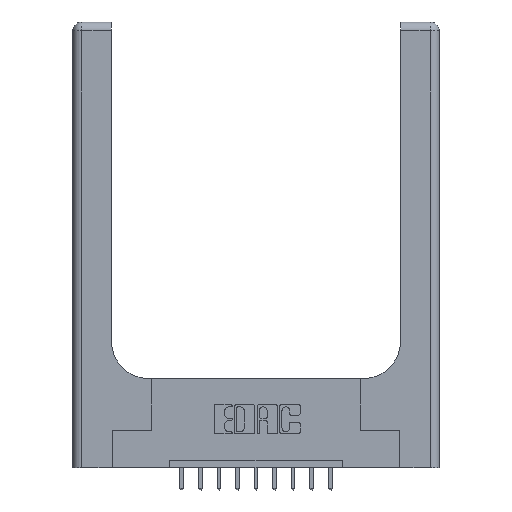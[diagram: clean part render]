
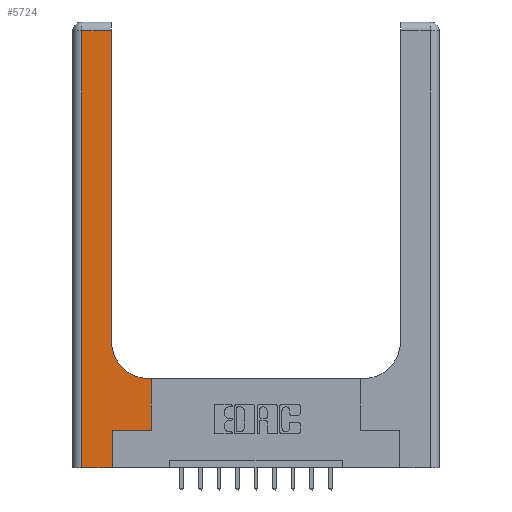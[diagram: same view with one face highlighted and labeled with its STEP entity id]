
A CAD part, top view. The second image highlights one B-rep face of the part: STEP entity #5724.
In plain terms, the highlighted planar face has unit normal (0, 0, 1).
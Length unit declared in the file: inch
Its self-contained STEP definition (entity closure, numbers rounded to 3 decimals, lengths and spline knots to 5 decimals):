
#124 = CARTESIAN_POINT ( 'NONE',  ( 0.528, 0.25, 0.37 ) ) ;
#149 = DIRECTION ( 'NONE',  ( 1., 0., 0. ) ) ;
#223 = CARTESIAN_POINT ( 'NONE',  ( 0.51, 0.85, 0.37 ) ) ;
#633 = DIRECTION ( 'NONE',  ( 0., 1., 0. ) ) ;
#662 = LINE ( 'NONE', #5479, #15247 ) ;
#711 = LINE ( 'NONE', #15052, #2263 ) ;
#1183 = LINE ( 'NONE', #14420, #14164 ) ;
#1320 = EDGE_CURVE ( 'NONE', #15670, #12019, #7495, .T. ) ;
#1458 = CARTESIAN_POINT ( 'NONE',  ( 0.26, 0.6, 0.37 ) ) ;
#1484 = VECTOR ( 'NONE', #2648, 39.37008 ) ;
#1538 = CARTESIAN_POINT ( 'NONE',  ( 0.265, 0.25, 0.37 ) ) ;
#1796 = ORIENTED_EDGE ( 'NONE', *, *, #11131, .T. ) ;
#2263 = VECTOR ( 'NONE', #633, 39.37008 ) ;
#2351 = EDGE_LOOP ( 'NONE', ( #15493, #11900, #12469, #4827, #13636, #3973, #2980, #12693, #1796 ) ) ;
#2383 = LINE ( 'NONE', #11051, #11143 ) ;
#2530 = VECTOR ( 'NONE', #12328, 39.37008 ) ;
#2648 = DIRECTION ( 'NONE',  ( 0., 1., 0. ) ) ;
#2891 = VERTEX_POINT ( 'NONE', #4877 ) ;
#2980 = ORIENTED_EDGE ( 'NONE', *, *, #1320, .T. ) ;
#3057 = DIRECTION ( 'NONE',  ( 0., 0., -1. ) ) ;
#3136 = DIRECTION ( 'NONE',  ( -1., 0., 0. ) ) ;
#3211 = FACE_OUTER_BOUND ( 'NONE', #2351, .T. ) ;
#3316 = EDGE_CURVE ( 'NONE', #12019, #2891, #11160, .T. ) ;
#3808 = AXIS2_PLACEMENT_3D ( 'NONE', #223, #11268, #149 ) ;
#3973 = ORIENTED_EDGE ( 'NONE', *, *, #5470, .T. ) ;
#4302 = CARTESIAN_POINT ( 'NONE',  ( 0.528, 0.25, 0.37 ) ) ;
#4585 = VERTEX_POINT ( 'NONE', #13779 ) ;
#4628 = VERTEX_POINT ( 'NONE', #14381 ) ;
#4827 = ORIENTED_EDGE ( 'NONE', *, *, #6338, .T. ) ;
#4877 = CARTESIAN_POINT ( 'NONE',  ( 0.51, 0.6, 0.37 ) ) ;
#5319 = CARTESIAN_POINT ( 'NONE',  ( 0.265, 0., 0.37 ) ) ;
#5470 = EDGE_CURVE ( 'NONE', #12850, #15670, #1183, .T. ) ;
#5479 = CARTESIAN_POINT ( 'NONE',  ( 0.06, 3., 0.37 ) ) ;
#5724 = ADVANCED_FACE ( 'NONE', ( #3211 ), #8146, .F. ) ;
#6338 = EDGE_CURVE ( 'NONE', #4628, #4585, #2383, .T. ) ;
#7105 = EDGE_CURVE ( 'NONE', #11960, #7735, #14673, .T. ) ;
#7495 = LINE ( 'NONE', #124, #1484 ) ;
#7673 = AXIS2_PLACEMENT_3D ( 'NONE', #11731, #3057, #3136 ) ;
#7735 = VERTEX_POINT ( 'NONE', #9636 ) ;
#7780 = CARTESIAN_POINT ( 'NONE',  ( 0.528, 0.6, 0.37 ) ) ;
#7884 = VECTOR ( 'NONE', #10253, 39.37008 ) ;
#8146 = PLANE ( 'NONE',  #7673 ) ;
#8441 = EDGE_CURVE ( 'NONE', #4585, #12850, #9130, .T. ) ;
#8839 = EDGE_CURVE ( 'NONE', #12697, #11960, #711, .T. ) ;
#9130 = LINE ( 'NONE', #5319, #7884 ) ;
#9636 = CARTESIAN_POINT ( 'NONE',  ( 0.06, 2.94, 0.37 ) ) ;
#9824 = DIRECTION ( 'NONE',  ( 1., 0., 0. ) ) ;
#10253 = DIRECTION ( 'NONE',  ( 0., 1., 0. ) ) ;
#10330 = DIRECTION ( 'NONE',  ( 0., -1., 0. ) ) ;
#11051 = CARTESIAN_POINT ( 'NONE',  ( 0., 0., 0.37 ) ) ;
#11131 = EDGE_CURVE ( 'NONE', #2891, #12697, #13231, .T. ) ;
#11143 = VECTOR ( 'NONE', #13429, 39.37008 ) ;
#11160 = LINE ( 'NONE', #1458, #14305 ) ;
#11268 = DIRECTION ( 'NONE',  ( 0., 0., -1. ) ) ;
#11731 = CARTESIAN_POINT ( 'NONE',  ( 0., 3., 0.37 ) ) ;
#11827 = EDGE_CURVE ( 'NONE', #7735, #4628, #662, .T. ) ;
#11900 = ORIENTED_EDGE ( 'NONE', *, *, #7105, .T. ) ;
#11960 = VERTEX_POINT ( 'NONE', #14977 ) ;
#12019 = VERTEX_POINT ( 'NONE', #7780 ) ;
#12328 = DIRECTION ( 'NONE',  ( -1., 0., 0. ) ) ;
#12354 = DIRECTION ( 'NONE',  ( -1., 0., 0. ) ) ;
#12407 = CARTESIAN_POINT ( 'NONE',  ( 0., 2.94, 0.37 ) ) ;
#12469 = ORIENTED_EDGE ( 'NONE', *, *, #11827, .T. ) ;
#12693 = ORIENTED_EDGE ( 'NONE', *, *, #3316, .T. ) ;
#12697 = VERTEX_POINT ( 'NONE', #15419 ) ;
#12850 = VERTEX_POINT ( 'NONE', #1538 ) ;
#13231 = CIRCLE ( 'NONE', #3808, 0.25 ) ;
#13429 = DIRECTION ( 'NONE',  ( 1., 0., 0. ) ) ;
#13636 = ORIENTED_EDGE ( 'NONE', *, *, #8441, .T. ) ;
#13779 = CARTESIAN_POINT ( 'NONE',  ( 0.265, 0., 0.37 ) ) ;
#14164 = VECTOR ( 'NONE', #9824, 39.37008 ) ;
#14305 = VECTOR ( 'NONE', #12354, 39.37008 ) ;
#14381 = CARTESIAN_POINT ( 'NONE',  ( 0.06, 0., 0.37 ) ) ;
#14420 = CARTESIAN_POINT ( 'NONE',  ( 0.265, 0.25, 0.37 ) ) ;
#14673 = LINE ( 'NONE', #12407, #2530 ) ;
#14977 = CARTESIAN_POINT ( 'NONE',  ( 0.26, 2.94, 0.37 ) ) ;
#15052 = CARTESIAN_POINT ( 'NONE',  ( 0.26, 3., 0.37 ) ) ;
#15247 = VECTOR ( 'NONE', #10330, 39.37008 ) ;
#15419 = CARTESIAN_POINT ( 'NONE',  ( 0.26, 0.85, 0.37 ) ) ;
#15493 = ORIENTED_EDGE ( 'NONE', *, *, #8839, .T. ) ;
#15670 = VERTEX_POINT ( 'NONE', #4302 ) ;
